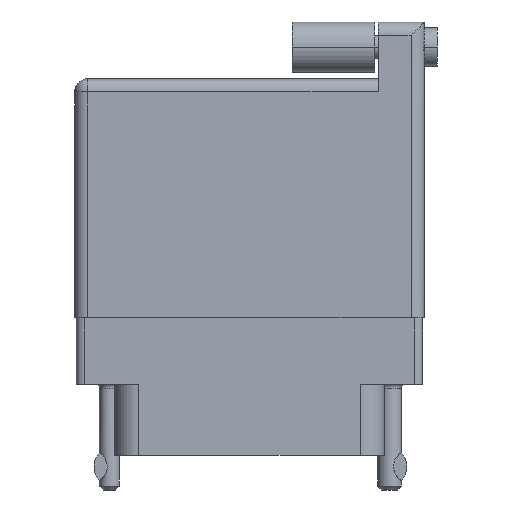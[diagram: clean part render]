
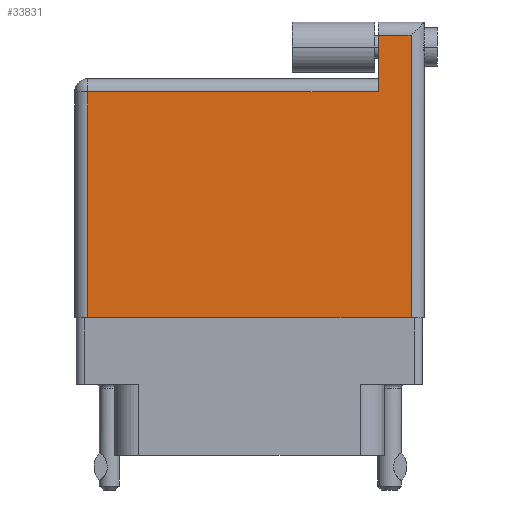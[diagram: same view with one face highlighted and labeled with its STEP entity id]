
A CAD part, front view. The second image highlights one B-rep face of the part: STEP entity #33831.
In plain terms, the highlighted face is planar.
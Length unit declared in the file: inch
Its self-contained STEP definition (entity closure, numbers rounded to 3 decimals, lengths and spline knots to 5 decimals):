
#142 = CARTESIAN_POINT ( 'NONE',  ( 1.275, 1.07, 0. ) ) ;
#933 = DIRECTION ( 'NONE',  ( 0., 0., -1. ) ) ;
#960 = CARTESIAN_POINT ( 'NONE',  ( 1.15, 1.07, 0. ) ) ;
#2054 = LINE ( 'NONE', #15072, #32449 ) ;
#3015 = CARTESIAN_POINT ( 'NONE',  ( 1.275, 1.12, 0. ) ) ;
#5025 = VERTEX_POINT ( 'NONE', #960 ) ;
#5732 = DIRECTION ( 'NONE',  ( 1., 0., 0. ) ) ;
#6882 = VERTEX_POINT ( 'NONE', #12270 ) ;
#8038 = DIRECTION ( 'NONE',  ( 0., -1., 0. ) ) ;
#9291 = AXIS2_PLACEMENT_3D ( 'NONE', #34494, #933, #31458 ) ;
#9917 = ORIENTED_EDGE ( 'NONE', *, *, #25128, .T. ) ;
#11549 = ORIENTED_EDGE ( 'NONE', *, *, #15386, .T. ) ;
#11892 = LINE ( 'NONE', #3015, #31332 ) ;
#11962 = VECTOR ( 'NONE', #31747, 39.37008 ) ;
#12270 = CARTESIAN_POINT ( 'NONE',  ( 0.05, 0.856, 0. ) ) ;
#12815 = LINE ( 'NONE', #20504, #11962 ) ;
#13881 = CARTESIAN_POINT ( 'NONE',  ( 0.05, 0., 0. ) ) ;
#15045 = ORIENTED_EDGE ( 'NONE', *, *, #25856, .T. ) ;
#15072 = CARTESIAN_POINT ( 'NONE',  ( 1.15, 1.12, 0. ) ) ;
#15386 = EDGE_CURVE ( 'NONE', #5025, #20127, #2054, .T. ) ;
#16818 = ORIENTED_EDGE ( 'NONE', *, *, #25423, .T. ) ;
#17362 = PLANE ( 'NONE',  #9291 ) ;
#18900 = VECTOR ( 'NONE', #5732, 39.37008 ) ;
#19160 = CARTESIAN_POINT ( 'NONE',  ( 0.05, 0., 0. ) ) ;
#19333 = VECTOR ( 'NONE', #32364, 39.37008 ) ;
#20127 = VERTEX_POINT ( 'NONE', #23973 ) ;
#20504 = CARTESIAN_POINT ( 'NONE',  ( 0., 0.856, 0. ) ) ;
#22019 = VERTEX_POINT ( 'NONE', #29009 ) ;
#22172 = EDGE_LOOP ( 'NONE', ( #16818, #24737, #32294, #11549, #9917, #15045 ) ) ;
#22329 = CARTESIAN_POINT ( 'NONE',  ( 0., 0., 0. ) ) ;
#23973 = CARTESIAN_POINT ( 'NONE',  ( 1.15, 0.856, 0. ) ) ;
#24136 = CARTESIAN_POINT ( 'NONE',  ( 0., 1.07, 0. ) ) ;
#24737 = ORIENTED_EDGE ( 'NONE', *, *, #26576, .T. ) ;
#25128 = EDGE_CURVE ( 'NONE', #20127, #6882, #12815, .T. ) ;
#25217 = EDGE_CURVE ( 'NONE', #34744, #5025, #33167, .T. ) ;
#25362 = VERTEX_POINT ( 'NONE', #13881 ) ;
#25423 = EDGE_CURVE ( 'NONE', #25362, #22019, #26243, .T. ) ;
#25818 = FACE_OUTER_BOUND ( 'NONE', #22172, .T. ) ;
#25856 = EDGE_CURVE ( 'NONE', #6882, #25362, #31407, .T. ) ;
#26066 = DIRECTION ( 'NONE',  ( 0., -1., 0. ) ) ;
#26243 = LINE ( 'NONE', #22329, #18900 ) ;
#26576 = EDGE_CURVE ( 'NONE', #22019, #34744, #11892, .T. ) ;
#29009 = CARTESIAN_POINT ( 'NONE',  ( 1.275, 0., 0. ) ) ;
#30113 = VECTOR ( 'NONE', #8038, 39.37008 ) ;
#30752 = DIRECTION ( 'NONE',  ( 0., 1., 0. ) ) ;
#31332 = VECTOR ( 'NONE', #30752, 39.37008 ) ;
#31407 = LINE ( 'NONE', #19160, #30113 ) ;
#31458 = DIRECTION ( 'NONE',  ( -1., 0., 0. ) ) ;
#31747 = DIRECTION ( 'NONE',  ( -1., 0., 0. ) ) ;
#32294 = ORIENTED_EDGE ( 'NONE', *, *, #25217, .T. ) ;
#32364 = DIRECTION ( 'NONE',  ( -1., 0., 0. ) ) ;
#32449 = VECTOR ( 'NONE', #26066, 39.37008 ) ;
#33167 = LINE ( 'NONE', #24136, #19333 ) ;
#33831 = ADVANCED_FACE ( 'NONE', ( #25818 ), #17362, .F. ) ;
#34494 = CARTESIAN_POINT ( 'NONE',  ( 0., 0.906, 0. ) ) ;
#34744 = VERTEX_POINT ( 'NONE', #142 ) ;
